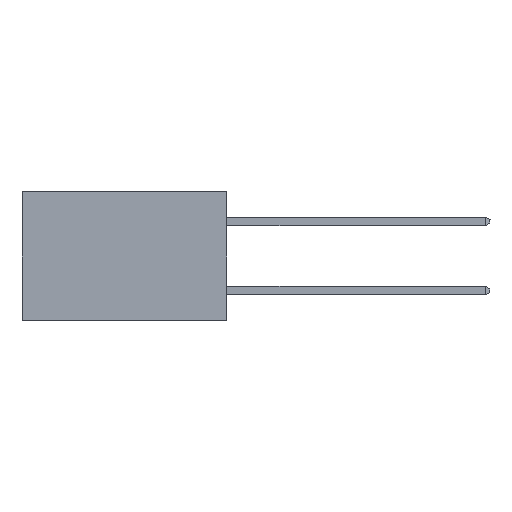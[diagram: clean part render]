
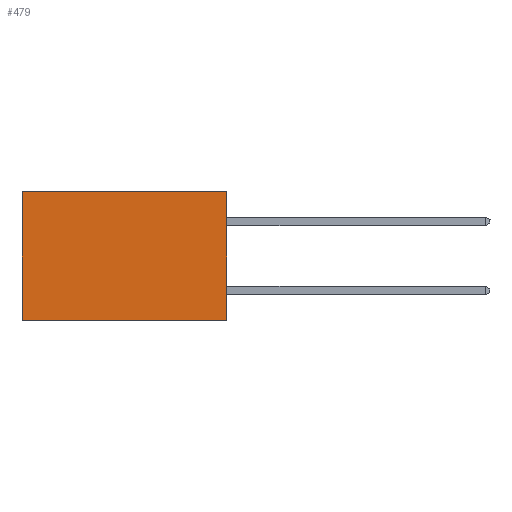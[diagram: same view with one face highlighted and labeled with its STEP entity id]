
A CAD part, left-side view. The second image highlights one B-rep face of the part: STEP entity #479.
In plain terms, the highlighted planar face has unit normal (-1, 0, 0).
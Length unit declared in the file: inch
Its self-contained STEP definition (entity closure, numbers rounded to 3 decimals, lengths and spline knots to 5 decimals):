
#81 = ORIENTED_EDGE ( 'NONE', *, *, #12190, .T. ) ;
#159 = VECTOR ( 'NONE', #9726, 39.37008 ) ;
#479 = ADVANCED_FACE ( 'NONE', ( #1749 ), #4807, .F. ) ;
#542 = LINE ( 'NONE', #3586, #159 ) ;
#1512 = DIRECTION ( 'NONE',  ( 0., 0., -1. ) ) ;
#1749 = FACE_OUTER_BOUND ( 'NONE', #8883, .T. ) ;
#2042 = CARTESIAN_POINT ( 'NONE',  ( 0.277, 0., -0.37 ) ) ;
#2365 = ORIENTED_EDGE ( 'NONE', *, *, #5352, .T. ) ;
#2722 = ORIENTED_EDGE ( 'NONE', *, *, #3555, .F. ) ;
#3555 = EDGE_CURVE ( 'NONE', #12339, #7867, #542, .T. ) ;
#3586 = CARTESIAN_POINT ( 'NONE',  ( 0.277, 0., -0.37 ) ) ;
#3818 = DIRECTION ( 'NONE',  ( 1., 0., 0. ) ) ;
#3961 = DIRECTION ( 'NONE',  ( 0., 1., 0. ) ) ;
#4439 = ORIENTED_EDGE ( 'NONE', *, *, #7245, .F. ) ;
#4545 = CARTESIAN_POINT ( 'NONE',  ( 0.277, 0.59, -0.37 ) ) ;
#4709 = DIRECTION ( 'NONE',  ( 0., 0., -1. ) ) ;
#4807 = PLANE ( 'NONE',  #11592 ) ;
#5352 = EDGE_CURVE ( 'NONE', #5922, #7867, #9239, .T. ) ;
#5597 = CARTESIAN_POINT ( 'NONE',  ( 0.277, 0.59, -0.37 ) ) ;
#5922 = VERTEX_POINT ( 'NONE', #15585 ) ;
#6495 = VERTEX_POINT ( 'NONE', #13112 ) ;
#6950 = VECTOR ( 'NONE', #13092, 39.37008 ) ;
#6986 = VECTOR ( 'NONE', #3961, 39.37008 ) ;
#7245 = EDGE_CURVE ( 'NONE', #6495, #12339, #10241, .T. ) ;
#7867 = VERTEX_POINT ( 'NONE', #5597 ) ;
#8883 = EDGE_LOOP ( 'NONE', ( #2365, #2722, #4439, #81 ) ) ;
#8939 = CARTESIAN_POINT ( 'NONE',  ( 0.277, 0., 0. ) ) ;
#9239 = LINE ( 'NONE', #4545, #9621 ) ;
#9562 = CARTESIAN_POINT ( 'NONE',  ( 0.277, 0., -0.37 ) ) ;
#9621 = VECTOR ( 'NONE', #4709, 39.37008 ) ;
#9726 = DIRECTION ( 'NONE',  ( 0., 1., 0. ) ) ;
#9936 = CARTESIAN_POINT ( 'NONE',  ( 0.277, 0., -0.37 ) ) ;
#10241 = LINE ( 'NONE', #9562, #6950 ) ;
#11592 = AXIS2_PLACEMENT_3D ( 'NONE', #9936, #3818, #1512 ) ;
#12190 = EDGE_CURVE ( 'NONE', #6495, #5922, #14060, .T. ) ;
#12339 = VERTEX_POINT ( 'NONE', #2042 ) ;
#13092 = DIRECTION ( 'NONE',  ( 0., 0., -1. ) ) ;
#13112 = CARTESIAN_POINT ( 'NONE',  ( 0.277, 0., 0. ) ) ;
#14060 = LINE ( 'NONE', #8939, #6986 ) ;
#15585 = CARTESIAN_POINT ( 'NONE',  ( 0.277, 0.59, 0. ) ) ;
